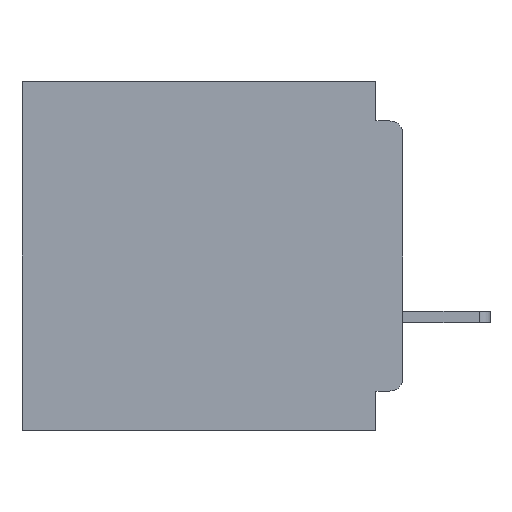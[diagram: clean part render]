
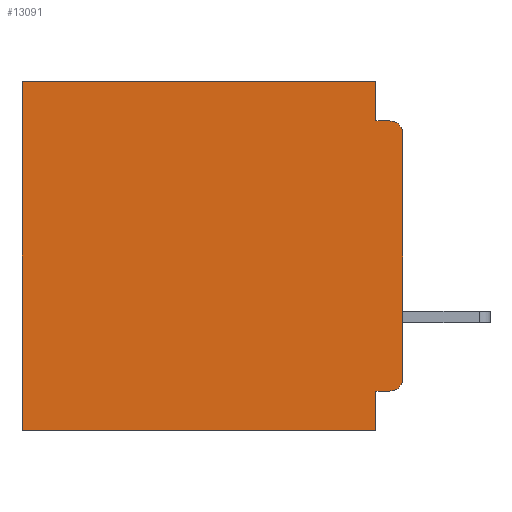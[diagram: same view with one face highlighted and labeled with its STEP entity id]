
A CAD part, left-side view. The second image highlights one B-rep face of the part: STEP entity #13091.
In plain terms, the highlighted planar face has unit normal (-1, 0, 0).
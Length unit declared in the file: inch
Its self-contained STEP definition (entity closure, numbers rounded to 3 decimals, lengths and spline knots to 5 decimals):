
#1503 = EDGE_CURVE ( 'NONE', #18672, #18138, #22288, .T. ) ;
#3158 = DIRECTION ( 'NONE',  ( 0., 0., -1. ) ) ;
#3281 = AXIS2_PLACEMENT_3D ( 'NONE', #24605, #58283, #29501 ) ;
#3406 = DIRECTION ( 'NONE',  ( 0., 0., -1. ) ) ;
#4663 = DIRECTION ( 'NONE',  ( 0., 0., -1. ) ) ;
#5099 = AXIS2_PLACEMENT_3D ( 'NONE', #20705, #54462, #25607 ) ;
#5102 = EDGE_LOOP ( 'NONE', ( #37310, #17233, #55464, #58335, #23724, #40287, #34982, #56264, #23548, #60612 ) ) ;
#8822 = CARTESIAN_POINT ( 'NONE',  ( 0.3, 0., -0.34 ) ) ;
#12357 = DIRECTION ( 'NONE',  ( 0., 1., 0. ) ) ;
#12360 = LINE ( 'NONE', #36604, #62282 ) ;
#12954 = EDGE_CURVE ( 'NONE', #35681, #57435, #58175, .T. ) ;
#13091 = ADVANCED_FACE ( 'NONE', ( #21927 ), #48153, .F. ) ;
#14985 = VERTEX_POINT ( 'NONE', #59574 ) ;
#15654 = VECTOR ( 'NONE', #54252, 39.37008 ) ;
#17233 = ORIENTED_EDGE ( 'NONE', *, *, #25379, .T. ) ;
#18138 = VERTEX_POINT ( 'NONE', #51397 ) ;
#18672 = VERTEX_POINT ( 'NONE', #59786 ) ;
#20705 = CARTESIAN_POINT ( 'NONE',  ( 0.3, 0.015, -0.06 ) ) ;
#21092 = DIRECTION ( 'NONE',  ( 0., 1., 0. ) ) ;
#21927 = FACE_OUTER_BOUND ( 'NONE', #5102, .T. ) ;
#22288 = LINE ( 'NONE', #59789, #59241 ) ;
#23548 = ORIENTED_EDGE ( 'NONE', *, *, #42845, .F. ) ;
#23724 = ORIENTED_EDGE ( 'NONE', *, *, #38160, .T. ) ;
#24426 = CARTESIAN_POINT ( 'NONE',  ( 0.3, 0., -0.045 ) ) ;
#24605 = CARTESIAN_POINT ( 'NONE',  ( 0.3, 0.015, -0.34 ) ) ;
#25010 = CARTESIAN_POINT ( 'NONE',  ( 0.3, 0., 0. ) ) ;
#25379 = EDGE_CURVE ( 'NONE', #35169, #14985, #41117, .T. ) ;
#25391 = LINE ( 'NONE', #24426, #36736 ) ;
#25607 = DIRECTION ( 'NONE',  ( 0., 0., -1. ) ) ;
#25651 = VERTEX_POINT ( 'NONE', #47053 ) ;
#25987 = CARTESIAN_POINT ( 'NONE',  ( 0.3, 0., -0.355 ) ) ;
#27583 = VECTOR ( 'NONE', #29892, 39.37008 ) ;
#28521 = VERTEX_POINT ( 'NONE', #60370 ) ;
#28584 = LINE ( 'NONE', #49400, #15654 ) ;
#29320 = DIRECTION ( 'NONE',  ( 0., -1., 0. ) ) ;
#29501 = DIRECTION ( 'NONE',  ( 0., 0., -1. ) ) ;
#29892 = DIRECTION ( 'NONE',  ( 0., 1., 0. ) ) ;
#30757 = EDGE_CURVE ( 'NONE', #35169, #39211, #28584, .T. ) ;
#32269 = LINE ( 'NONE', #25987, #43549 ) ;
#32739 = EDGE_CURVE ( 'NONE', #40596, #57435, #12360, .T. ) ;
#33203 = CARTESIAN_POINT ( 'NONE',  ( 0.3, 0.437, -0.4 ) ) ;
#33835 = DIRECTION ( 'NONE',  ( 1., 0., 0. ) ) ;
#34982 = ORIENTED_EDGE ( 'NONE', *, *, #32739, .F. ) ;
#35169 = VERTEX_POINT ( 'NONE', #48569 ) ;
#35681 = VERTEX_POINT ( 'NONE', #48074 ) ;
#36604 = CARTESIAN_POINT ( 'NONE',  ( 0.3, 0., -0.4 ) ) ;
#36675 = VECTOR ( 'NONE', #57443, 39.37008 ) ;
#36736 = VECTOR ( 'NONE', #29320, 39.37008 ) ;
#37310 = ORIENTED_EDGE ( 'NONE', *, *, #30757, .F. ) ;
#37541 = EDGE_CURVE ( 'NONE', #18138, #14985, #25391, .T. ) ;
#37972 = EDGE_CURVE ( 'NONE', #25651, #40596, #62247, .T. ) ;
#38160 = EDGE_CURVE ( 'NONE', #18672, #35681, #41923, .T. ) ;
#39211 = VERTEX_POINT ( 'NONE', #8822 ) ;
#40287 = ORIENTED_EDGE ( 'NONE', *, *, #12954, .T. ) ;
#40596 = VERTEX_POINT ( 'NONE', #46838 ) ;
#41117 = CIRCLE ( 'NONE', #5099, 0.015 ) ;
#41470 = EDGE_CURVE ( 'NONE', #28521, #39211, #48340, .T. ) ;
#41923 = LINE ( 'NONE', #25010, #27583 ) ;
#42076 = CARTESIAN_POINT ( 'NONE',  ( 0.3, 0.437, -0.4 ) ) ;
#42093 = CARTESIAN_POINT ( 'NONE',  ( 0.3, 0.031, -0.4 ) ) ;
#42845 = EDGE_CURVE ( 'NONE', #28521, #25651, #32269, .T. ) ;
#43549 = VECTOR ( 'NONE', #21092, 39.37008 ) ;
#46838 = CARTESIAN_POINT ( 'NONE',  ( 0.3, 0.031, -0.4 ) ) ;
#47053 = CARTESIAN_POINT ( 'NONE',  ( 0.3, 0.031, -0.355 ) ) ;
#48074 = CARTESIAN_POINT ( 'NONE',  ( 0.3, 0.437, 0. ) ) ;
#48153 = PLANE ( 'NONE',  #49315 ) ;
#48340 = CIRCLE ( 'NONE', #3281, 0.015 ) ;
#48569 = CARTESIAN_POINT ( 'NONE',  ( 0.3, 0., -0.06 ) ) ;
#49315 = AXIS2_PLACEMENT_3D ( 'NONE', #62648, #33835, #4663 ) ;
#49400 = CARTESIAN_POINT ( 'NONE',  ( 0.3, 0., -0.4 ) ) ;
#51397 = CARTESIAN_POINT ( 'NONE',  ( 0.3, 0.031, -0.045 ) ) ;
#54252 = DIRECTION ( 'NONE',  ( 0., 0., -1. ) ) ;
#54462 = DIRECTION ( 'NONE',  ( -1., 0., 0. ) ) ;
#55464 = ORIENTED_EDGE ( 'NONE', *, *, #37541, .F. ) ;
#56264 = ORIENTED_EDGE ( 'NONE', *, *, #37972, .F. ) ;
#56677 = VECTOR ( 'NONE', #3406, 39.37008 ) ;
#57435 = VERTEX_POINT ( 'NONE', #33203 ) ;
#57443 = DIRECTION ( 'NONE',  ( 0., 0., -1. ) ) ;
#58175 = LINE ( 'NONE', #42076, #56677 ) ;
#58283 = DIRECTION ( 'NONE',  ( -1., 0., 0. ) ) ;
#58335 = ORIENTED_EDGE ( 'NONE', *, *, #1503, .F. ) ;
#59241 = VECTOR ( 'NONE', #3158, 39.37008 ) ;
#59574 = CARTESIAN_POINT ( 'NONE',  ( 0.3, 0.015, -0.045 ) ) ;
#59786 = CARTESIAN_POINT ( 'NONE',  ( 0.3, 0.031, 0. ) ) ;
#59789 = CARTESIAN_POINT ( 'NONE',  ( 0.3, 0.031, 0. ) ) ;
#60370 = CARTESIAN_POINT ( 'NONE',  ( 0.3, 0.015, -0.355 ) ) ;
#60612 = ORIENTED_EDGE ( 'NONE', *, *, #41470, .T. ) ;
#62247 = LINE ( 'NONE', #42093, #36675 ) ;
#62282 = VECTOR ( 'NONE', #12357, 39.37008 ) ;
#62648 = CARTESIAN_POINT ( 'NONE',  ( 0.3, 0., -0.4 ) ) ;
